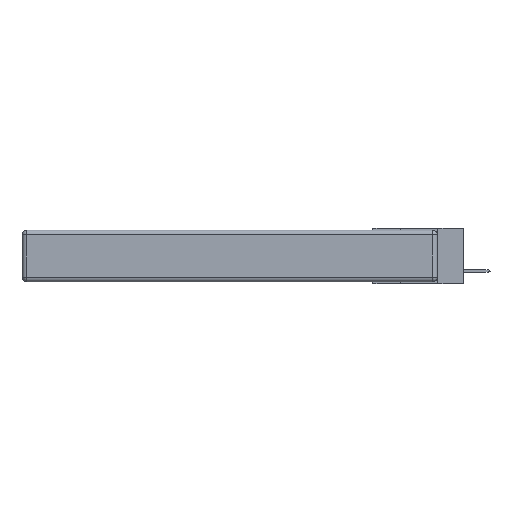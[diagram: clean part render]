
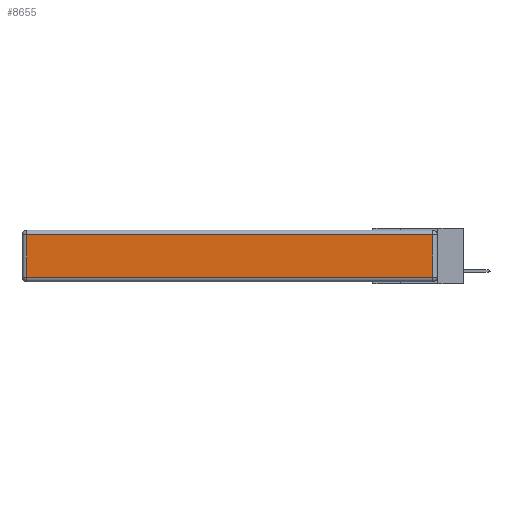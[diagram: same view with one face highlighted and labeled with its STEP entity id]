
A CAD part, left-side view. The second image highlights one B-rep face of the part: STEP entity #8655.
In plain terms, the highlighted planar face has unit normal (-1, 0, 0).
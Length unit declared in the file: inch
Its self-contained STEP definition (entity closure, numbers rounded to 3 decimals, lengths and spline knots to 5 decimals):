
#418 = VERTEX_POINT ( 'NONE', #1645 ) ;
#718 = PLANE ( 'NONE',  #1663 ) ;
#1501 = LINE ( 'NONE', #11784, #4141 ) ;
#1645 = CARTESIAN_POINT ( 'NONE',  ( 0., 0.03, -0.313 ) ) ;
#1663 = AXIS2_PLACEMENT_3D ( 'NONE', #6356, #4133, #14248 ) ;
#2238 = ORIENTED_EDGE ( 'NONE', *, *, #13641, .T. ) ;
#2375 = EDGE_CURVE ( 'NONE', #11046, #8871, #14193, .T. ) ;
#3306 = ORIENTED_EDGE ( 'NONE', *, *, #11440, .T. ) ;
#4043 = EDGE_CURVE ( 'NONE', #418, #4780, #12290, .T. ) ;
#4133 = DIRECTION ( 'NONE',  ( -1., 0., 0. ) ) ;
#4141 = VECTOR ( 'NONE', #10693, 39.37008 ) ;
#4678 = CARTESIAN_POINT ( 'NONE',  ( 0., 0.03, -0.03 ) ) ;
#4749 = CARTESIAN_POINT ( 'NONE',  ( 0., 2.72, -0.343 ) ) ;
#4780 = VERTEX_POINT ( 'NONE', #4678 ) ;
#5128 = ORIENTED_EDGE ( 'NONE', *, *, #2375, .T. ) ;
#5624 = VECTOR ( 'NONE', #6543, 39.37008 ) ;
#6263 = VECTOR ( 'NONE', #7017, 39.37008 ) ;
#6356 = CARTESIAN_POINT ( 'NONE',  ( 0., 0., -0.343 ) ) ;
#6543 = DIRECTION ( 'NONE',  ( 0., 0., 1. ) ) ;
#7017 = DIRECTION ( 'NONE',  ( 0., 1., 0. ) ) ;
#7620 = CARTESIAN_POINT ( 'NONE',  ( 0., 0.03, -0.343 ) ) ;
#7884 = EDGE_LOOP ( 'NONE', ( #3306, #9743, #2238, #5128 ) ) ;
#8655 = ADVANCED_FACE ( 'NONE', ( #10691 ), #718, .T. ) ;
#8871 = VERTEX_POINT ( 'NONE', #10087 ) ;
#9743 = ORIENTED_EDGE ( 'NONE', *, *, #4043, .T. ) ;
#10087 = CARTESIAN_POINT ( 'NONE',  ( 0., 2.72, -0.313 ) ) ;
#10489 = DIRECTION ( 'NONE',  ( 0., 0., -1. ) ) ;
#10691 = FACE_OUTER_BOUND ( 'NONE', #7884, .T. ) ;
#10693 = DIRECTION ( 'NONE',  ( 0., -1., 0. ) ) ;
#11046 = VERTEX_POINT ( 'NONE', #11119 ) ;
#11119 = CARTESIAN_POINT ( 'NONE',  ( 0., 2.72, -0.03 ) ) ;
#11374 = CARTESIAN_POINT ( 'NONE',  ( 0., 2.75, -0.03 ) ) ;
#11440 = EDGE_CURVE ( 'NONE', #8871, #418, #1501, .T. ) ;
#11784 = CARTESIAN_POINT ( 'NONE',  ( 0., 0., -0.313 ) ) ;
#12290 = LINE ( 'NONE', #7620, #5624 ) ;
#12565 = LINE ( 'NONE', #11374, #6263 ) ;
#13641 = EDGE_CURVE ( 'NONE', #4780, #11046, #12565, .T. ) ;
#13831 = VECTOR ( 'NONE', #10489, 39.37008 ) ;
#14193 = LINE ( 'NONE', #4749, #13831 ) ;
#14248 = DIRECTION ( 'NONE',  ( 0., 0., 1. ) ) ;
